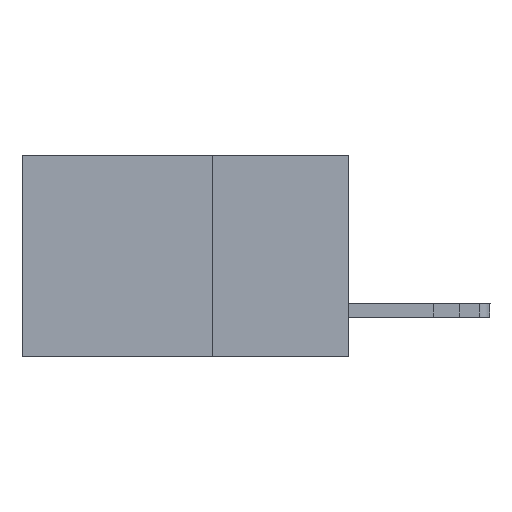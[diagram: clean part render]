
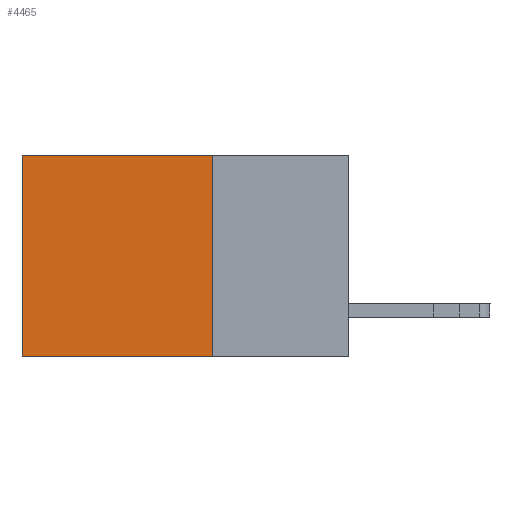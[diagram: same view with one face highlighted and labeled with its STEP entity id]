
A CAD part, left-side view. The second image highlights one B-rep face of the part: STEP entity #4465.
In plain terms, the highlighted planar face has unit normal (-1, 0, 0).
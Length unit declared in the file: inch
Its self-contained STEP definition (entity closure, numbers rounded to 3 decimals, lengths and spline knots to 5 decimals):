
#651 = CARTESIAN_POINT ( 'NONE',  ( 0.2615, 0.25, -0.37 ) ) ;
#692 = ORIENTED_EDGE ( 'NONE', *, *, #6570, .F. ) ;
#2820 = EDGE_LOOP ( 'NONE', ( #5185, #4627, #692, #9606 ) ) ;
#3103 = DIRECTION ( 'NONE',  ( 0., 1., 0. ) ) ;
#3149 = VERTEX_POINT ( 'NONE', #6777 ) ;
#3302 = DIRECTION ( 'NONE',  ( 1., 0., 0. ) ) ;
#3446 = CARTESIAN_POINT ( 'NONE',  ( 0.2615, 0.25, -0.37 ) ) ;
#4465 = ADVANCED_FACE ( 'NONE', ( #6890 ), #11374, .F. ) ;
#4627 = ORIENTED_EDGE ( 'NONE', *, *, #5275, .F. ) ;
#4879 = CARTESIAN_POINT ( 'NONE',  ( 0.2615, 0.25, 0. ) ) ;
#4955 = CARTESIAN_POINT ( 'NONE',  ( 0.2615, 0.25, 0. ) ) ;
#5159 = CARTESIAN_POINT ( 'NONE',  ( 0.2615, 0.6, -0.37 ) ) ;
#5185 = ORIENTED_EDGE ( 'NONE', *, *, #5335, .T. ) ;
#5275 = EDGE_CURVE ( 'NONE', #6630, #8796, #8516, .T. ) ;
#5335 = EDGE_CURVE ( 'NONE', #3149, #8796, #8632, .T. ) ;
#5761 = VECTOR ( 'NONE', #8406, 39.37008 ) ;
#5875 = LINE ( 'NONE', #4879, #5761 ) ;
#6260 = VECTOR ( 'NONE', #9641, 39.37008 ) ;
#6570 = EDGE_CURVE ( 'NONE', #9117, #6630, #7876, .T. ) ;
#6630 = VERTEX_POINT ( 'NONE', #7982 ) ;
#6777 = CARTESIAN_POINT ( 'NONE',  ( 0.2615, 0.6, 0. ) ) ;
#6890 = FACE_OUTER_BOUND ( 'NONE', #2820, .T. ) ;
#7295 = VECTOR ( 'NONE', #3103, 39.37008 ) ;
#7515 = VECTOR ( 'NONE', #9584, 39.37008 ) ;
#7876 = LINE ( 'NONE', #3446, #6260 ) ;
#7968 = AXIS2_PLACEMENT_3D ( 'NONE', #651, #3302, #9662 ) ;
#7982 = CARTESIAN_POINT ( 'NONE',  ( 0.2615, 0.25, -0.37 ) ) ;
#8406 = DIRECTION ( 'NONE',  ( 0., 1., 0. ) ) ;
#8516 = LINE ( 'NONE', #11176, #7295 ) ;
#8632 = LINE ( 'NONE', #5159, #7515 ) ;
#8796 = VERTEX_POINT ( 'NONE', #10619 ) ;
#9117 = VERTEX_POINT ( 'NONE', #4955 ) ;
#9584 = DIRECTION ( 'NONE',  ( 0., 0., -1. ) ) ;
#9606 = ORIENTED_EDGE ( 'NONE', *, *, #10055, .T. ) ;
#9641 = DIRECTION ( 'NONE',  ( 0., 0., -1. ) ) ;
#9662 = DIRECTION ( 'NONE',  ( 0., 0., -1. ) ) ;
#10055 = EDGE_CURVE ( 'NONE', #9117, #3149, #5875, .T. ) ;
#10619 = CARTESIAN_POINT ( 'NONE',  ( 0.2615, 0.6, -0.37 ) ) ;
#11176 = CARTESIAN_POINT ( 'NONE',  ( 0.2615, 0.25, -0.37 ) ) ;
#11374 = PLANE ( 'NONE',  #7968 ) ;
